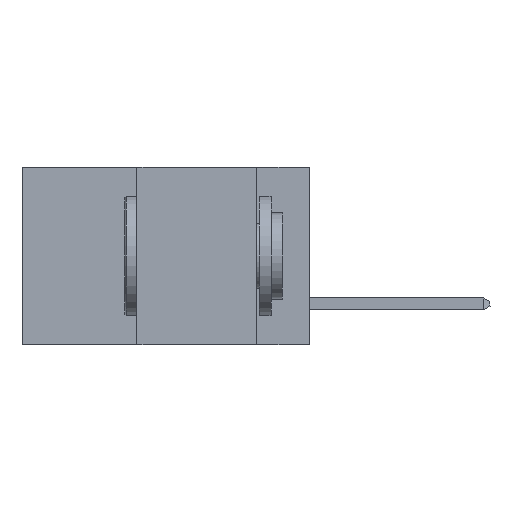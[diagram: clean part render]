
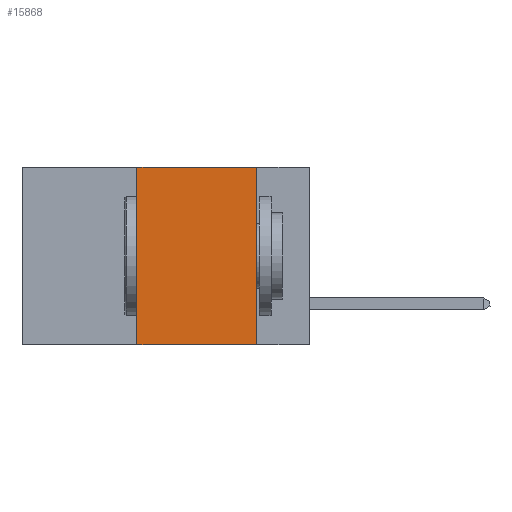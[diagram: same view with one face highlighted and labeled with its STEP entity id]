
A CAD part, left-side view. The second image highlights one B-rep face of the part: STEP entity #15868.
In plain terms, the highlighted planar face has unit normal (-1, 0, 0).
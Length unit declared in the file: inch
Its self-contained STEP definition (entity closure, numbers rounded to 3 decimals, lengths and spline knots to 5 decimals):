
#2368 = CARTESIAN_POINT ( 'NONE',  ( 0., 0.11, 0. ) ) ;
#2410 = DIRECTION ( 'NONE',  ( 0., 0., -1. ) ) ;
#2930 = EDGE_CURVE ( 'NONE', #5895, #8388, #23140, .T. ) ;
#3496 = VERTEX_POINT ( 'NONE', #7084 ) ;
#4561 = CARTESIAN_POINT ( 'NONE',  ( 0., 0.36, 0. ) ) ;
#5394 = CARTESIAN_POINT ( 'NONE',  ( 0., 0.6, 0. ) ) ;
#5895 = VERTEX_POINT ( 'NONE', #2368 ) ;
#7084 = CARTESIAN_POINT ( 'NONE',  ( 0., 0.36, -0.37 ) ) ;
#7426 = DIRECTION ( 'NONE',  ( 0., -1., 0. ) ) ;
#7617 = VECTOR ( 'NONE', #8108, 39.37008 ) ;
#8108 = DIRECTION ( 'NONE',  ( 0., 0., -1. ) ) ;
#8111 = CARTESIAN_POINT ( 'NONE',  ( 0., 0.36, 0. ) ) ;
#8339 = ORIENTED_EDGE ( 'NONE', *, *, #15217, .T. ) ;
#8388 = VERTEX_POINT ( 'NONE', #8754 ) ;
#8404 = LINE ( 'NONE', #5394, #18047 ) ;
#8561 = PLANE ( 'NONE',  #20207 ) ;
#8754 = CARTESIAN_POINT ( 'NONE',  ( 0., 0.11, -0.37 ) ) ;
#8790 = EDGE_CURVE ( 'NONE', #3496, #17181, #22084, .T. ) ;
#9663 = CARTESIAN_POINT ( 'NONE',  ( 0., 0.11, 0. ) ) ;
#12207 = CARTESIAN_POINT ( 'NONE',  ( 0., 0.6, -0.37 ) ) ;
#12428 = CARTESIAN_POINT ( 'NONE',  ( 0., 0.6, 0. ) ) ;
#14356 = DIRECTION ( 'NONE',  ( 1., 0., 0. ) ) ;
#14875 = LINE ( 'NONE', #12207, #19442 ) ;
#15217 = EDGE_CURVE ( 'NONE', #3496, #8388, #14875, .T. ) ;
#15778 = DIRECTION ( 'NONE',  ( 0., 0., 1. ) ) ;
#15868 = ADVANCED_FACE ( 'NONE', ( #19698 ), #8561, .F. ) ;
#16872 = VECTOR ( 'NONE', #15778, 39.37008 ) ;
#17181 = VERTEX_POINT ( 'NONE', #4561 ) ;
#17981 = ORIENTED_EDGE ( 'NONE', *, *, #24210, .F. ) ;
#18047 = VECTOR ( 'NONE', #7426, 39.37008 ) ;
#19442 = VECTOR ( 'NONE', #23801, 39.37008 ) ;
#19698 = FACE_OUTER_BOUND ( 'NONE', #20231, .T. ) ;
#20207 = AXIS2_PLACEMENT_3D ( 'NONE', #12428, #14356, #2410 ) ;
#20231 = EDGE_LOOP ( 'NONE', ( #21972, #17981, #23209, #8339 ) ) ;
#21972 = ORIENTED_EDGE ( 'NONE', *, *, #2930, .F. ) ;
#22084 = LINE ( 'NONE', #8111, #16872 ) ;
#23140 = LINE ( 'NONE', #9663, #7617 ) ;
#23209 = ORIENTED_EDGE ( 'NONE', *, *, #8790, .F. ) ;
#23801 = DIRECTION ( 'NONE',  ( 0., -1., 0. ) ) ;
#24210 = EDGE_CURVE ( 'NONE', #17181, #5895, #8404, .T. ) ;
